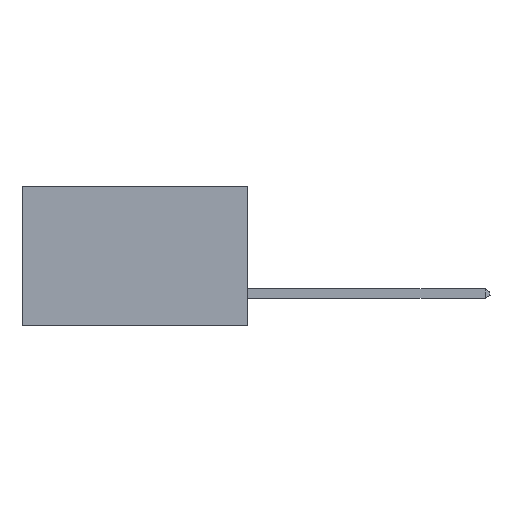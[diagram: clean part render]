
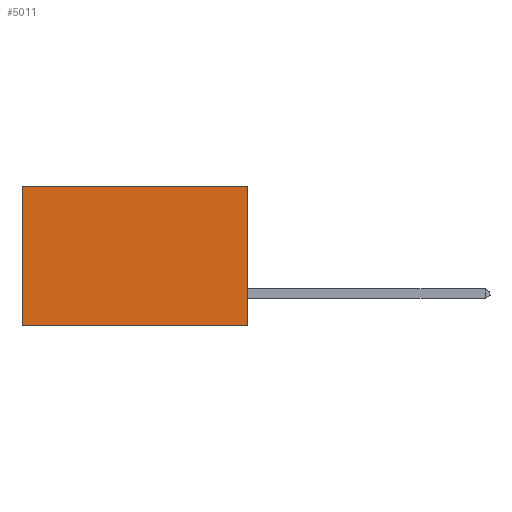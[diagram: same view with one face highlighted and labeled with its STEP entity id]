
A CAD part, left-side view. The second image highlights one B-rep face of the part: STEP entity #5011.
In plain terms, the highlighted planar face has unit normal (-1, 0, 0).
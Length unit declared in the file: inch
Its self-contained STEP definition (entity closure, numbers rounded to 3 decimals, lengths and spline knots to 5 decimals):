
#209 = EDGE_CURVE ( 'NONE', #1118, #3926, #10846, .T. ) ;
#637 = EDGE_LOOP ( 'NONE', ( #10772, #14090, #9223, #4932 ) ) ;
#961 = EDGE_CURVE ( 'NONE', #10267, #1118, #9133, .T. ) ;
#1118 = VERTEX_POINT ( 'NONE', #15800 ) ;
#1763 = CARTESIAN_POINT ( 'NONE',  ( 0.298, 0., -0.37 ) ) ;
#1826 = DIRECTION ( 'NONE',  ( 0., 1., 0. ) ) ;
#3926 = VERTEX_POINT ( 'NONE', #14685 ) ;
#4175 = EDGE_CURVE ( 'NONE', #10267, #11467, #14981, .T. ) ;
#4932 = ORIENTED_EDGE ( 'NONE', *, *, #4175, .T. ) ;
#5011 = ADVANCED_FACE ( 'NONE', ( #11801 ), #14348, .F. ) ;
#6245 = LINE ( 'NONE', #11168, #13826 ) ;
#7267 = VECTOR ( 'NONE', #1826, 39.37008 ) ;
#7638 = DIRECTION ( 'NONE',  ( 0., 0., -1. ) ) ;
#8606 = DIRECTION ( 'NONE',  ( 0., 0., -1. ) ) ;
#9133 = LINE ( 'NONE', #16474, #11422 ) ;
#9223 = ORIENTED_EDGE ( 'NONE', *, *, #961, .F. ) ;
#9461 = CARTESIAN_POINT ( 'NONE',  ( 0.298, 0., 0. ) ) ;
#10267 = VERTEX_POINT ( 'NONE', #10517 ) ;
#10327 = AXIS2_PLACEMENT_3D ( 'NONE', #11625, #15674, #7638 ) ;
#10517 = CARTESIAN_POINT ( 'NONE',  ( 0.298, 0., 0. ) ) ;
#10772 = ORIENTED_EDGE ( 'NONE', *, *, #12659, .T. ) ;
#10846 = LINE ( 'NONE', #1763, #7267 ) ;
#11168 = CARTESIAN_POINT ( 'NONE',  ( 0.298, 0.6, 0. ) ) ;
#11329 = DIRECTION ( 'NONE',  ( 0., 0., -1. ) ) ;
#11404 = VECTOR ( 'NONE', #16222, 39.37008 ) ;
#11422 = VECTOR ( 'NONE', #8606, 39.37008 ) ;
#11467 = VERTEX_POINT ( 'NONE', #13604 ) ;
#11625 = CARTESIAN_POINT ( 'NONE',  ( 0.298, 0., 0. ) ) ;
#11801 = FACE_OUTER_BOUND ( 'NONE', #637, .T. ) ;
#12659 = EDGE_CURVE ( 'NONE', #11467, #3926, #6245, .T. ) ;
#13604 = CARTESIAN_POINT ( 'NONE',  ( 0.298, 0.6, 0. ) ) ;
#13826 = VECTOR ( 'NONE', #11329, 39.37008 ) ;
#14090 = ORIENTED_EDGE ( 'NONE', *, *, #209, .F. ) ;
#14348 = PLANE ( 'NONE',  #10327 ) ;
#14685 = CARTESIAN_POINT ( 'NONE',  ( 0.298, 0.6, -0.37 ) ) ;
#14981 = LINE ( 'NONE', #9461, #11404 ) ;
#15674 = DIRECTION ( 'NONE',  ( 1., 0., 0. ) ) ;
#15800 = CARTESIAN_POINT ( 'NONE',  ( 0.298, 0., -0.37 ) ) ;
#16222 = DIRECTION ( 'NONE',  ( 0., 1., 0. ) ) ;
#16474 = CARTESIAN_POINT ( 'NONE',  ( 0.298, 0., 0. ) ) ;
